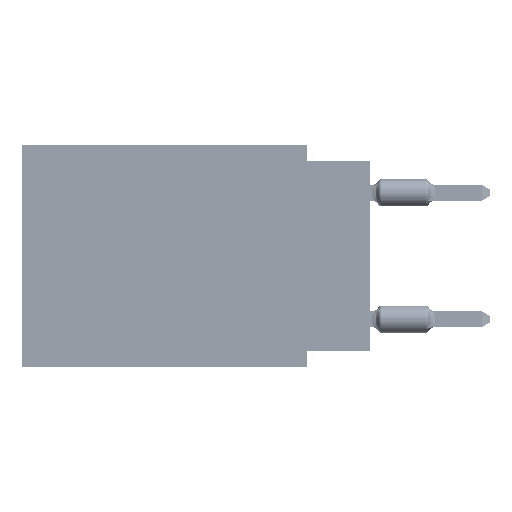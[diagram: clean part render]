
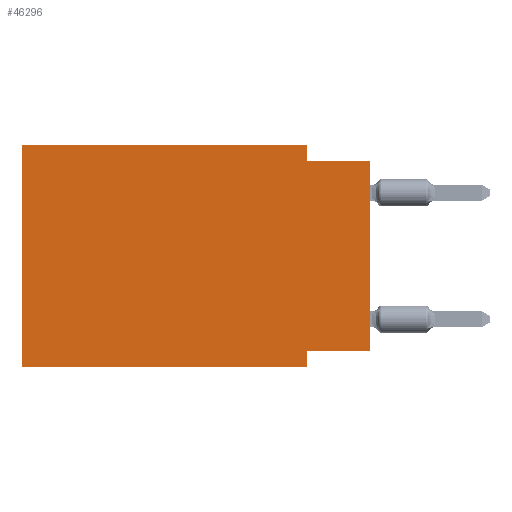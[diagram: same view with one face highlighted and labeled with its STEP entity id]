
A CAD part, left-side view. The second image highlights one B-rep face of the part: STEP entity #46296.
In plain terms, the highlighted planar face has unit normal (-1, 0, 0).
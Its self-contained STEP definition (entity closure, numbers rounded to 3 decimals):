
#2001 = CARTESIAN_POINT ( 'NONE',  ( 0., 0., -8.255 ) ) ;
#2120 = VERTEX_POINT ( 'NONE', #12121 ) ;
#3254 = DIRECTION ( 'NONE',  ( 0., 0., -1. ) ) ;
#3448 = VECTOR ( 'NONE', #4323, 1000. ) ;
#3927 = DIRECTION ( 'NONE',  ( 0., -1., 0. ) ) ;
#4323 = DIRECTION ( 'NONE',  ( 0., -1., 0. ) ) ;
#4964 = CARTESIAN_POINT ( 'NONE',  ( 0., 0., -8.255 ) ) ;
#6621 = EDGE_CURVE ( 'NONE', #61806, #2120, #21455, .T. ) ;
#6653 = VERTEX_POINT ( 'NONE', #28073 ) ;
#7672 = VECTOR ( 'NONE', #46313, 1000. ) ;
#8089 = DIRECTION ( 'NONE',  ( 0., 0., 1. ) ) ;
#9046 = CARTESIAN_POINT ( 'NONE',  ( 0., 2.54, 0. ) ) ;
#9061 = CARTESIAN_POINT ( 'NONE',  ( 0., 0., -0.635 ) ) ;
#9349 = PLANE ( 'NONE',  #25146 ) ;
#12121 = CARTESIAN_POINT ( 'NONE',  ( 0., 2.54, -0.635 ) ) ;
#13472 = LINE ( 'NONE', #45347, #63553 ) ;
#14981 = ORIENTED_EDGE ( 'NONE', *, *, #27790, .F. ) ;
#15326 = VERTEX_POINT ( 'NONE', #35794 ) ;
#16062 = DIRECTION ( 'NONE',  ( 0., 1., 0. ) ) ;
#16205 = ORIENTED_EDGE ( 'NONE', *, *, #17757, .F. ) ;
#17757 = EDGE_CURVE ( 'NONE', #47328, #6653, #47519, .T. ) ;
#18214 = CARTESIAN_POINT ( 'NONE',  ( 0., 0., 0. ) ) ;
#19065 = CARTESIAN_POINT ( 'NONE',  ( 0., 2.54, 0. ) ) ;
#19750 = EDGE_CURVE ( 'NONE', #47328, #57371, #80728, .T. ) ;
#21249 = CARTESIAN_POINT ( 'NONE',  ( 0., 13.97, 0. ) ) ;
#21455 = LINE ( 'NONE', #9046, #7672 ) ;
#21852 = CARTESIAN_POINT ( 'NONE',  ( 0., 2.54, -8.89 ) ) ;
#22107 = DIRECTION ( 'NONE',  ( 0., -1., 0. ) ) ;
#25146 = AXIS2_PLACEMENT_3D ( 'NONE', #34595, #65232, #71852 ) ;
#26911 = ORIENTED_EDGE ( 'NONE', *, *, #37915, .T. ) ;
#27790 = EDGE_CURVE ( 'NONE', #6653, #15326, #78584, .T. ) ;
#28073 = CARTESIAN_POINT ( 'NONE',  ( 0., 2.54, -8.255 ) ) ;
#33318 = EDGE_CURVE ( 'NONE', #2120, #57371, #53562, .T. ) ;
#34378 = VECTOR ( 'NONE', #22107, 1000. ) ;
#34452 = EDGE_CURVE ( 'NONE', #54042, #51994, #13472, .T. ) ;
#34520 = EDGE_CURVE ( 'NONE', #51994, #61806, #66418, .T. ) ;
#34595 = CARTESIAN_POINT ( 'NONE',  ( 0., 13.97, 0. ) ) ;
#34956 = LINE ( 'NONE', #54416, #3448 ) ;
#35794 = CARTESIAN_POINT ( 'NONE',  ( 0., 2.54, -8.89 ) ) ;
#37915 = EDGE_CURVE ( 'NONE', #54042, #15326, #34956, .T. ) ;
#38660 = ORIENTED_EDGE ( 'NONE', *, *, #19750, .T. ) ;
#45068 = VECTOR ( 'NONE', #3927, 1000. ) ;
#45347 = CARTESIAN_POINT ( 'NONE',  ( 0., 13.97, 0. ) ) ;
#46296 = ADVANCED_FACE ( 'NONE', ( #72672 ), #9349, .F. ) ;
#46313 = DIRECTION ( 'NONE',  ( 0., 0., -1. ) ) ;
#47111 = EDGE_LOOP ( 'NONE', ( #38660, #56641, #70117, #61053, #81408, #26911, #14981, #16205 ) ) ;
#47328 = VERTEX_POINT ( 'NONE', #4964 ) ;
#47519 = LINE ( 'NONE', #2001, #67076 ) ;
#51994 = VERTEX_POINT ( 'NONE', #21249 ) ;
#53171 = CARTESIAN_POINT ( 'NONE',  ( 0., 0., -0.635 ) ) ;
#53562 = LINE ( 'NONE', #53171, #34378 ) ;
#54042 = VERTEX_POINT ( 'NONE', #64542 ) ;
#54416 = CARTESIAN_POINT ( 'NONE',  ( 0., 13.97, -8.89 ) ) ;
#55057 = VECTOR ( 'NONE', #3254, 1000. ) ;
#56641 = ORIENTED_EDGE ( 'NONE', *, *, #33318, .F. ) ;
#57371 = VERTEX_POINT ( 'NONE', #9061 ) ;
#61053 = ORIENTED_EDGE ( 'NONE', *, *, #34520, .F. ) ;
#61806 = VERTEX_POINT ( 'NONE', #19065 ) ;
#63553 = VECTOR ( 'NONE', #8089, 1000. ) ;
#64542 = CARTESIAN_POINT ( 'NONE',  ( 0., 13.97, -8.89 ) ) ;
#65232 = DIRECTION ( 'NONE',  ( 1., 0., 0. ) ) ;
#66418 = LINE ( 'NONE', #66817, #45068 ) ;
#66817 = CARTESIAN_POINT ( 'NONE',  ( 0., 13.97, 0. ) ) ;
#67076 = VECTOR ( 'NONE', #16062, 1000. ) ;
#69780 = VECTOR ( 'NONE', #74497, 1000. ) ;
#70117 = ORIENTED_EDGE ( 'NONE', *, *, #6621, .F. ) ;
#71852 = DIRECTION ( 'NONE',  ( 0., 0., -1. ) ) ;
#72672 = FACE_OUTER_BOUND ( 'NONE', #47111, .T. ) ;
#74497 = DIRECTION ( 'NONE',  ( 0., 0., 1. ) ) ;
#78584 = LINE ( 'NONE', #21852, #55057 ) ;
#80728 = LINE ( 'NONE', #18214, #69780 ) ;
#81408 = ORIENTED_EDGE ( 'NONE', *, *, #34452, .F. ) ;
